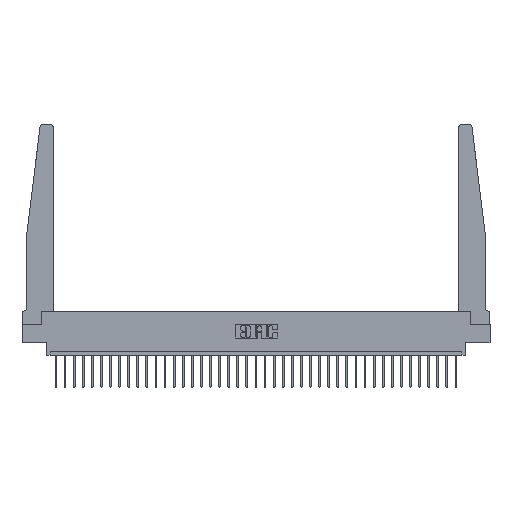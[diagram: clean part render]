
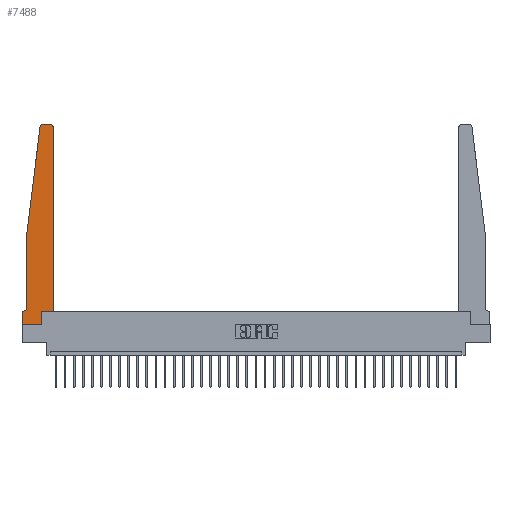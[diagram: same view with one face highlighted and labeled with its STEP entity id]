
A CAD part, top view. The second image highlights one B-rep face of the part: STEP entity #7488.
In plain terms, the highlighted planar face has unit normal (0, 0, 1).
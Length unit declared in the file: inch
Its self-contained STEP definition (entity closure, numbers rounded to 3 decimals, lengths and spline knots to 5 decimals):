
#5 = CARTESIAN_POINT ( 'NONE',  ( 0.015, 0.2375, 0.37 ) ) ;
#505 = ORIENTED_EDGE ( 'NONE', *, *, #4521, .T. ) ;
#1053 = LINE ( 'NONE', #9925, #31991 ) ;
#1503 = DIRECTION ( 'NONE',  ( -0.122, -0.992, 0. ) ) ;
#1706 = VECTOR ( 'NONE', #1503, 39.37008 ) ;
#2255 = AXIS2_PLACEMENT_3D ( 'NONE', #24297, #29237, #16683 ) ;
#2379 = EDGE_CURVE ( 'NONE', #17509, #6911, #27880, .T. ) ;
#2489 = DIRECTION ( 'NONE',  ( 0., 1., 0. ) ) ;
#2512 = ORIENTED_EDGE ( 'NONE', *, *, #4048, .T. ) ;
#2664 = ORIENTED_EDGE ( 'NONE', *, *, #21302, .T. ) ;
#2735 = CIRCLE ( 'NONE', #15432, 0.05 ) ;
#4048 = EDGE_CURVE ( 'NONE', #22515, #10418, #2735, .T. ) ;
#4521 = EDGE_CURVE ( 'NONE', #19764, #23207, #20360, .T. ) ;
#4840 = CARTESIAN_POINT ( 'NONE',  ( 0.24675, 2.72367, 0.37 ) ) ;
#4937 = VERTEX_POINT ( 'NONE', #12900 ) ;
#5062 = EDGE_CURVE ( 'NONE', #27921, #19764, #9720, .T. ) ;
#5111 = CARTESIAN_POINT ( 'NONE',  ( 0.27653, 2.75, 0.37 ) ) ;
#5432 = CARTESIAN_POINT ( 'NONE',  ( 0.015, 0.1875, 0.37 ) ) ;
#5704 = CARTESIAN_POINT ( 'NONE',  ( 0.2605, 0.18, 0.37 ) ) ;
#5784 = EDGE_CURVE ( 'NONE', #18266, #17509, #22974, .T. ) ;
#5870 = AXIS2_PLACEMENT_3D ( 'NONE', #19753, #7230, #9754 ) ;
#6268 = LINE ( 'NONE', #14793, #25855 ) ;
#6716 = CARTESIAN_POINT ( 'NONE',  ( 0., 0., 0.37 ) ) ;
#6812 = DIRECTION ( 'NONE',  ( 0., -1., 0. ) ) ;
#6911 = VERTEX_POINT ( 'NONE', #5704 ) ;
#7230 = DIRECTION ( 'NONE',  ( 0., 0., 1. ) ) ;
#7488 = ADVANCED_FACE ( 'NONE', ( #28000 ), #20221, .T. ) ;
#7883 = DIRECTION ( 'NONE',  ( 1., 0., 0. ) ) ;
#7894 = DIRECTION ( 'NONE',  ( 1., 0., 0. ) ) ;
#8125 = CARTESIAN_POINT ( 'NONE',  ( 0., 0.1875, 0.37 ) ) ;
#8722 = ORIENTED_EDGE ( 'NONE', *, *, #9870, .T. ) ;
#9251 = VERTEX_POINT ( 'NONE', #4840 ) ;
#9720 = CIRCLE ( 'NONE', #2255, 0.03 ) ;
#9754 = DIRECTION ( 'NONE',  ( 1., 0., 0. ) ) ;
#9870 = EDGE_CURVE ( 'NONE', #23207, #9251, #23925, .T. ) ;
#9925 = CARTESIAN_POINT ( 'NONE',  ( 0.425, 0.18, 0.37 ) ) ;
#10356 = VERTEX_POINT ( 'NONE', #15071 ) ;
#10418 = VERTEX_POINT ( 'NONE', #5432 ) ;
#10664 = DIRECTION ( 'NONE',  ( -1., 0., 0. ) ) ;
#11471 = VECTOR ( 'NONE', #21034, 39.37008 ) ;
#11747 = DIRECTION ( 'NONE',  ( -1., 0., 0. ) ) ;
#12075 = ORIENTED_EDGE ( 'NONE', *, *, #5062, .T. ) ;
#12081 = VERTEX_POINT ( 'NONE', #19276 ) ;
#12133 = CARTESIAN_POINT ( 'NONE',  ( 0.395, 2.75, 0.37 ) ) ;
#12518 = EDGE_CURVE ( 'NONE', #12081, #22515, #29082, .T. ) ;
#12585 = AXIS2_PLACEMENT_3D ( 'NONE', #8125, #27723, #7894 ) ;
#12900 = CARTESIAN_POINT ( 'NONE',  ( 0.425, 0.18, 0.37 ) ) ;
#13317 = CARTESIAN_POINT ( 'NONE',  ( 0.065, 1.25, 0.37 ) ) ;
#14079 = VECTOR ( 'NONE', #10664, 39.37008 ) ;
#14249 = ORIENTED_EDGE ( 'NONE', *, *, #27350, .T. ) ;
#14271 = CARTESIAN_POINT ( 'NONE',  ( 0.2605, 0., 0.37 ) ) ;
#14434 = CARTESIAN_POINT ( 'NONE',  ( 0.425, 2.72, 0.37 ) ) ;
#14793 = CARTESIAN_POINT ( 'NONE',  ( 0., 0., 0.37 ) ) ;
#15071 = CARTESIAN_POINT ( 'NONE',  ( 0., 0.1875, 0.37 ) ) ;
#15073 = EDGE_CURVE ( 'NONE', #6911, #4937, #22679, .T. ) ;
#15432 = AXIS2_PLACEMENT_3D ( 'NONE', #5, #29001, #11747 ) ;
#15749 = ORIENTED_EDGE ( 'NONE', *, *, #15073, .T. ) ;
#16287 = CARTESIAN_POINT ( 'NONE',  ( 0.065, 1.25, 0.37 ) ) ;
#16471 = VECTOR ( 'NONE', #21310, 39.37008 ) ;
#16683 = DIRECTION ( 'NONE',  ( 1., 0., 0. ) ) ;
#17509 = VERTEX_POINT ( 'NONE', #14271 ) ;
#18266 = VERTEX_POINT ( 'NONE', #6716 ) ;
#18531 = CARTESIAN_POINT ( 'NONE',  ( 0.2605, 0.18, 0.37 ) ) ;
#19276 = CARTESIAN_POINT ( 'NONE',  ( 0.065, 1.25, 0.37 ) ) ;
#19753 = CARTESIAN_POINT ( 'NONE',  ( 0.27653, 2.72, 0.37 ) ) ;
#19764 = VERTEX_POINT ( 'NONE', #12133 ) ;
#19868 = ORIENTED_EDGE ( 'NONE', *, *, #25254, .T. ) ;
#20221 = PLANE ( 'NONE',  #12585 ) ;
#20360 = LINE ( 'NONE', #26053, #14079 ) ;
#20414 = ORIENTED_EDGE ( 'NONE', *, *, #12518, .T. ) ;
#20415 = CARTESIAN_POINT ( 'NONE',  ( 0., 0., 0.37 ) ) ;
#21034 = DIRECTION ( 'NONE',  ( 0., 1., 0. ) ) ;
#21277 = LINE ( 'NONE', #16287, #1706 ) ;
#21302 = EDGE_CURVE ( 'NONE', #10418, #10356, #23880, .T. ) ;
#21310 = DIRECTION ( 'NONE',  ( -1., 0., 0. ) ) ;
#21844 = ORIENTED_EDGE ( 'NONE', *, *, #29748, .T. ) ;
#21927 = DIRECTION ( 'NONE',  ( 1., 0., 0. ) ) ;
#22058 = VECTOR ( 'NONE', #28177, 39.37008 ) ;
#22515 = VERTEX_POINT ( 'NONE', #23927 ) ;
#22679 = LINE ( 'NONE', #31782, #23442 ) ;
#22974 = LINE ( 'NONE', #20415, #23740 ) ;
#23207 = VERTEX_POINT ( 'NONE', #5111 ) ;
#23442 = VECTOR ( 'NONE', #21927, 39.37008 ) ;
#23740 = VECTOR ( 'NONE', #7883, 39.37008 ) ;
#23880 = LINE ( 'NONE', #28518, #16471 ) ;
#23925 = CIRCLE ( 'NONE', #5870, 0.03 ) ;
#23927 = CARTESIAN_POINT ( 'NONE',  ( 0.065, 0.2375, 0.37 ) ) ;
#24297 = CARTESIAN_POINT ( 'NONE',  ( 0.395, 2.72, 0.37 ) ) ;
#24449 = ORIENTED_EDGE ( 'NONE', *, *, #5784, .T. ) ;
#25254 = EDGE_CURVE ( 'NONE', #9251, #12081, #21277, .T. ) ;
#25855 = VECTOR ( 'NONE', #6812, 39.37008 ) ;
#26053 = CARTESIAN_POINT ( 'NONE',  ( 0.25, 2.75, 0.37 ) ) ;
#27171 = ORIENTED_EDGE ( 'NONE', *, *, #2379, .T. ) ;
#27350 = EDGE_CURVE ( 'NONE', #10356, #18266, #6268, .T. ) ;
#27723 = DIRECTION ( 'NONE',  ( 0., 0., 1. ) ) ;
#27880 = LINE ( 'NONE', #18531, #11471 ) ;
#27921 = VERTEX_POINT ( 'NONE', #14434 ) ;
#28000 = FACE_OUTER_BOUND ( 'NONE', #30241, .T. ) ;
#28177 = DIRECTION ( 'NONE',  ( 0., -1., 0. ) ) ;
#28518 = CARTESIAN_POINT ( 'NONE',  ( 0.065, 0.1875, 0.37 ) ) ;
#29001 = DIRECTION ( 'NONE',  ( 0., 0., -1. ) ) ;
#29082 = LINE ( 'NONE', #13317, #22058 ) ;
#29237 = DIRECTION ( 'NONE',  ( 0., 0., 1. ) ) ;
#29748 = EDGE_CURVE ( 'NONE', #4937, #27921, #1053, .T. ) ;
#30241 = EDGE_LOOP ( 'NONE', ( #505, #8722, #19868, #20414, #2512, #2664, #14249, #24449, #27171, #15749, #21844, #12075 ) ) ;
#31782 = CARTESIAN_POINT ( 'NONE',  ( 0.425, 0.18, 0.37 ) ) ;
#31991 = VECTOR ( 'NONE', #2489, 39.37008 ) ;
